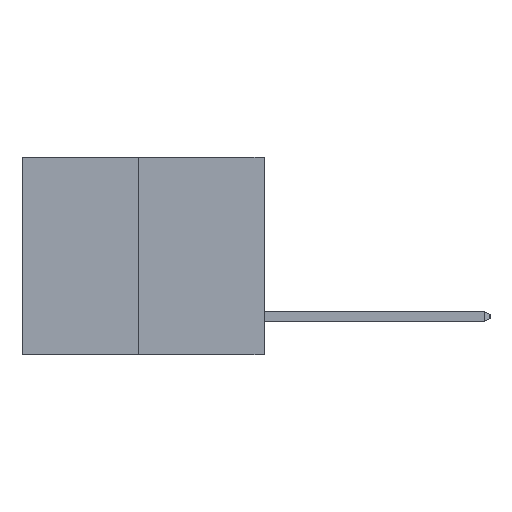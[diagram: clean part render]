
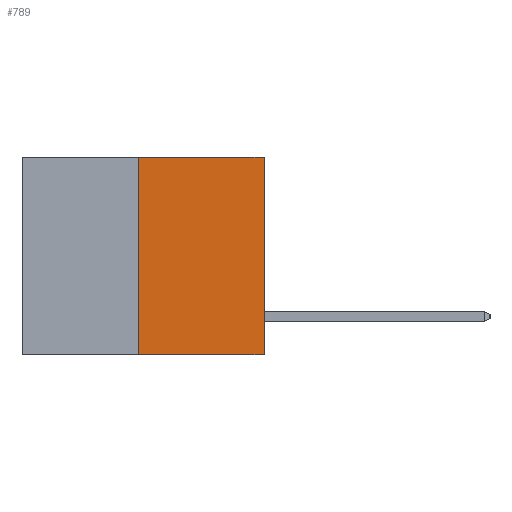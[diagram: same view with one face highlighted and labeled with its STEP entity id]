
A CAD part, left-side view. The second image highlights one B-rep face of the part: STEP entity #789.
In plain terms, the highlighted planar face has unit normal (-1, 0, 0).
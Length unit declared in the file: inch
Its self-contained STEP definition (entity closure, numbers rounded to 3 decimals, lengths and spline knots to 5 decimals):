
#219 = CARTESIAN_POINT ( 'NONE',  ( 0., 0.312, -0.49 ) ) ;
#721 = EDGE_CURVE ( 'NONE', #11982, #9285, #4893, .T. ) ;
#789 = ADVANCED_FACE ( 'NONE', ( #1494 ), #10524, .F. ) ;
#1282 = DIRECTION ( 'NONE',  ( 1., 0., 0. ) ) ;
#1290 = EDGE_CURVE ( 'NONE', #7048, #11502, #8929, .T. ) ;
#1494 = FACE_OUTER_BOUND ( 'NONE', #11476, .T. ) ;
#2089 = VECTOR ( 'NONE', #13291, 39.37008 ) ;
#2158 = VECTOR ( 'NONE', #8201, 39.37008 ) ;
#2232 = CARTESIAN_POINT ( 'NONE',  ( 0., 0.6, 0. ) ) ;
#2428 = ORIENTED_EDGE ( 'NONE', *, *, #1290, .T. ) ;
#2553 = ORIENTED_EDGE ( 'NONE', *, *, #6523, .T. ) ;
#2862 = AXIS2_PLACEMENT_3D ( 'NONE', #2232, #1282, #12650 ) ;
#3419 = LINE ( 'NONE', #12438, #4051 ) ;
#3726 = ORIENTED_EDGE ( 'NONE', *, *, #11419, .F. ) ;
#4051 = VECTOR ( 'NONE', #8229, 39.37008 ) ;
#4433 = CARTESIAN_POINT ( 'NONE',  ( 0., 0., 0. ) ) ;
#4830 = LINE ( 'NONE', #10235, #2089 ) ;
#4893 = LINE ( 'NONE', #10298, #2158 ) ;
#5537 = VECTOR ( 'NONE', #13112, 39.37008 ) ;
#6024 = CARTESIAN_POINT ( 'NONE',  ( 0., 0.6, -0.49 ) ) ;
#6523 = EDGE_CURVE ( 'NONE', #11502, #9285, #4830, .T. ) ;
#6868 = CARTESIAN_POINT ( 'NONE',  ( 0., 0.312, 0. ) ) ;
#7048 = VERTEX_POINT ( 'NONE', #219 ) ;
#8201 = DIRECTION ( 'NONE',  ( 0., -1., 0. ) ) ;
#8229 = DIRECTION ( 'NONE',  ( 0., 0., 1. ) ) ;
#8925 = ORIENTED_EDGE ( 'NONE', *, *, #721, .F. ) ;
#8929 = LINE ( 'NONE', #6024, #5537 ) ;
#9285 = VERTEX_POINT ( 'NONE', #4433 ) ;
#10235 = CARTESIAN_POINT ( 'NONE',  ( 0., 0., 0. ) ) ;
#10298 = CARTESIAN_POINT ( 'NONE',  ( 0., 0.6, 0. ) ) ;
#10524 = PLANE ( 'NONE',  #2862 ) ;
#11419 = EDGE_CURVE ( 'NONE', #7048, #11982, #3419, .T. ) ;
#11476 = EDGE_LOOP ( 'NONE', ( #3726, #2428, #2553, #8925 ) ) ;
#11502 = VERTEX_POINT ( 'NONE', #12679 ) ;
#11982 = VERTEX_POINT ( 'NONE', #6868 ) ;
#12438 = CARTESIAN_POINT ( 'NONE',  ( 0., 0.312, -0.49 ) ) ;
#12650 = DIRECTION ( 'NONE',  ( 0., 0., -1. ) ) ;
#12679 = CARTESIAN_POINT ( 'NONE',  ( 0., 0., -0.49 ) ) ;
#13112 = DIRECTION ( 'NONE',  ( 0., -1., 0. ) ) ;
#13291 = DIRECTION ( 'NONE',  ( 0., 0., 1. ) ) ;
